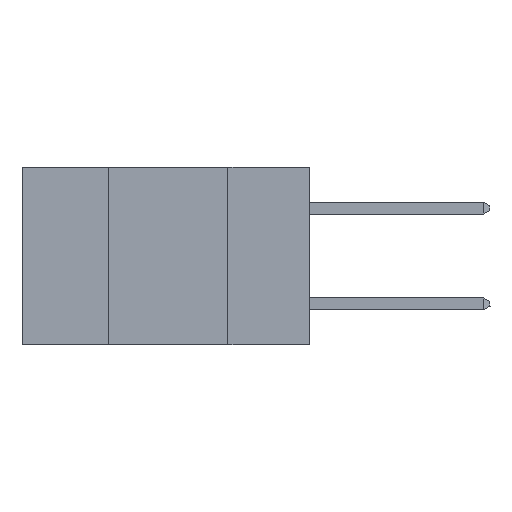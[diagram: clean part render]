
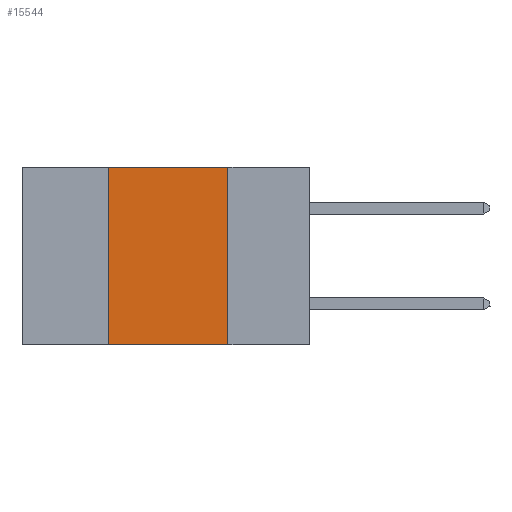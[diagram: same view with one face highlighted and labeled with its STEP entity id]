
A CAD part, left-side view. The second image highlights one B-rep face of the part: STEP entity #15544.
In plain terms, the highlighted planar face has unit normal (-1, 0, 0).
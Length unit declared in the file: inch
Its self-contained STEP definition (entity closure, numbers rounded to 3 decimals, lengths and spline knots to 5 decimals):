
#218 = LINE ( 'NONE', #16488, #10939 ) ;
#349 = ORIENTED_EDGE ( 'NONE', *, *, #12053, .T. ) ;
#382 = VECTOR ( 'NONE', #15533, 39.37008 ) ;
#759 = CARTESIAN_POINT ( 'NONE',  ( 0., 0.17, 0. ) ) ;
#1126 = ORIENTED_EDGE ( 'NONE', *, *, #12914, .F. ) ;
#1705 = DIRECTION ( 'NONE',  ( 1., 0., 0. ) ) ;
#2368 = VECTOR ( 'NONE', #3470, 39.37008 ) ;
#2569 = CARTESIAN_POINT ( 'NONE',  ( 0., 0.6, -0.37 ) ) ;
#2939 = EDGE_LOOP ( 'NONE', ( #6825, #10100, #1126, #349 ) ) ;
#3470 = DIRECTION ( 'NONE',  ( 0., -1., 0. ) ) ;
#4828 = VERTEX_POINT ( 'NONE', #6832 ) ;
#5594 = CARTESIAN_POINT ( 'NONE',  ( 0., 0.17, -0.37 ) ) ;
#5985 = DIRECTION ( 'NONE',  ( 0., 0., 1. ) ) ;
#5993 = PLANE ( 'NONE',  #16833 ) ;
#6354 = CARTESIAN_POINT ( 'NONE',  ( 0., 0.17, 0. ) ) ;
#6762 = VERTEX_POINT ( 'NONE', #5594 ) ;
#6825 = ORIENTED_EDGE ( 'NONE', *, *, #13746, .F. ) ;
#6832 = CARTESIAN_POINT ( 'NONE',  ( 0., 0.42, 0. ) ) ;
#7016 = VECTOR ( 'NONE', #13504, 39.37008 ) ;
#7288 = FACE_OUTER_BOUND ( 'NONE', #2939, .T. ) ;
#7620 = VERTEX_POINT ( 'NONE', #12701 ) ;
#7863 = VERTEX_POINT ( 'NONE', #759 ) ;
#8312 = LINE ( 'NONE', #2569, #7016 ) ;
#10061 = CARTESIAN_POINT ( 'NONE',  ( 0., 0.6, 0. ) ) ;
#10100 = ORIENTED_EDGE ( 'NONE', *, *, #10759, .F. ) ;
#10759 = EDGE_CURVE ( 'NONE', #4828, #7863, #17042, .T. ) ;
#10939 = VECTOR ( 'NONE', #5985, 39.37008 ) ;
#11395 = DIRECTION ( 'NONE',  ( 0., 0., -1. ) ) ;
#12053 = EDGE_CURVE ( 'NONE', #7620, #6762, #8312, .T. ) ;
#12701 = CARTESIAN_POINT ( 'NONE',  ( 0., 0.42, -0.37 ) ) ;
#12914 = EDGE_CURVE ( 'NONE', #7620, #4828, #218, .T. ) ;
#13504 = DIRECTION ( 'NONE',  ( 0., -1., 0. ) ) ;
#13746 = EDGE_CURVE ( 'NONE', #7863, #6762, #14086, .T. ) ;
#14086 = LINE ( 'NONE', #6354, #382 ) ;
#14151 = CARTESIAN_POINT ( 'NONE',  ( 0., 0.6, 0. ) ) ;
#15533 = DIRECTION ( 'NONE',  ( 0., 0., -1. ) ) ;
#15544 = ADVANCED_FACE ( 'NONE', ( #7288 ), #5993, .F. ) ;
#16488 = CARTESIAN_POINT ( 'NONE',  ( 0., 0.42, 0. ) ) ;
#16833 = AXIS2_PLACEMENT_3D ( 'NONE', #10061, #1705, #11395 ) ;
#17042 = LINE ( 'NONE', #14151, #2368 ) ;
